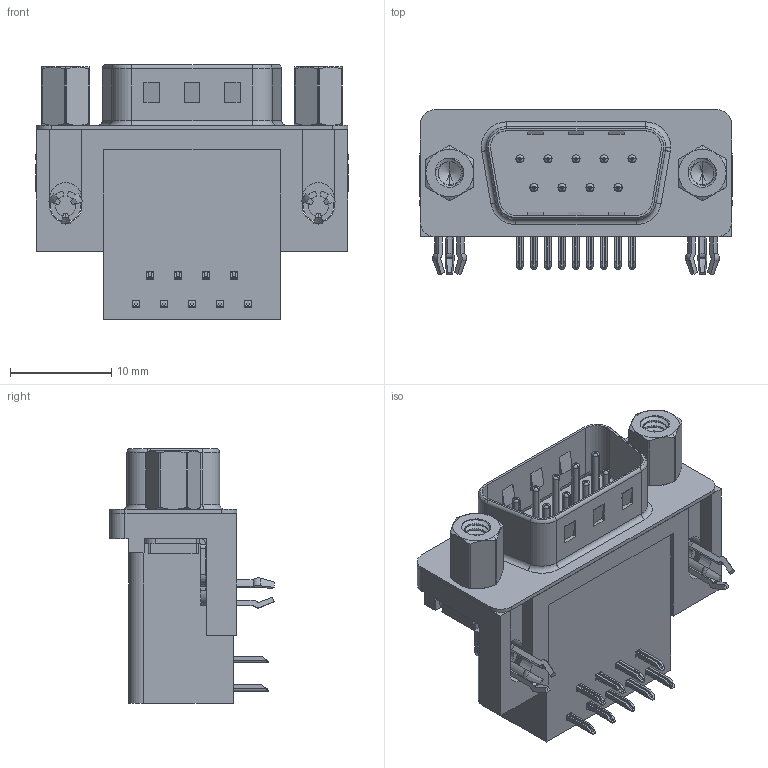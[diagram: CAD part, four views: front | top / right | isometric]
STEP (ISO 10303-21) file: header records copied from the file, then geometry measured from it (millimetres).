
FILE_DESCRIPTION (( 'STEP AP203' ), '1' );
FILE_NAME ('625-009-262-543.STEP', '2018-11-05T20:22:24', ( '' ), ( '' ), 'SwSTEP 2.0', 'SolidWorks 2016', '' );
FILE_SCHEMA (( 'CONFIG_CONTROL_DESIGN' ));
Length unit declared in the file: millimetre
Products named in the file (8): 625 4-40 Threaded Rivet; 625 4-40 Hex Standoff 5; 625-009-262-543; 625 Housing_9 Socket; 625 Shell_9 Socket; 625 Contact Bottom; 625 Contact Top; 625 3 Prong Board Lock
Assembly tree (17 placements, depth 2):
  625-009-262-543
    625 Housing_9 Socket
    625 Shell_9 Socket
    625 Contact Bottom  x4
    625 Contact Top  x5
    625 3 Prong Board Lock  x2
    625 4-40 Threaded Rivet  x2
    625 4-40 Hex Standoff 5  x2
Bounding box: 30.89 x 16.25 x 25.16 mm (x, y, z)
Volume: 4697.3 mm3; surface area: 5495.1 mm2
Topology: 17 solids, 17 shells, 1223 faces, 3141 edges, 1977 vertices
Faces by surface type: plane 633, cylinder 395, torus 109, cone 68, bspline 18
Entity records: 22884 total; most frequent: CARTESIAN_POINT 7701, DIRECTION 2971, ORIENTED_EDGE 2954, EDGE_CURVE 1477, AXIS2_PLACEMENT_3D 1047, VERTEX_POINT 946, VECTOR 877, LINE 877
